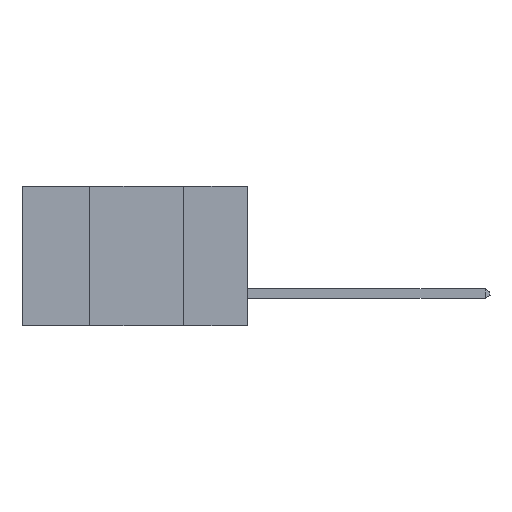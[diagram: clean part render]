
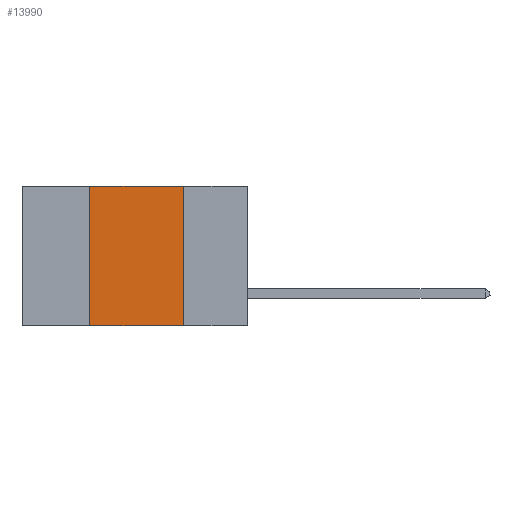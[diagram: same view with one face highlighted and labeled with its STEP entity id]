
A CAD part, left-side view. The second image highlights one B-rep face of the part: STEP entity #13990.
In plain terms, the highlighted planar face has unit normal (-1, 0, 0).
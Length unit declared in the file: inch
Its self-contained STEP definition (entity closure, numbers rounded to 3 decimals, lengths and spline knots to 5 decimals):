
#1462 = DIRECTION ( 'NONE',  ( 0., 0., -1. ) ) ;
#1663 = CARTESIAN_POINT ( 'NONE',  ( 0., 0.6, 0. ) ) ;
#2090 = DIRECTION ( 'NONE',  ( 0., -1., 0. ) ) ;
#2326 = VERTEX_POINT ( 'NONE', #18614 ) ;
#2506 = ORIENTED_EDGE ( 'NONE', *, *, #29750, .F. ) ;
#3122 = EDGE_CURVE ( 'NONE', #29241, #19191, #11850, .T. ) ;
#3670 = DIRECTION ( 'NONE',  ( 1., 0., 0. ) ) ;
#6490 = CARTESIAN_POINT ( 'NONE',  ( 0., 0.17, -0.37 ) ) ;
#7082 = LINE ( 'NONE', #9182, #16496 ) ;
#9182 = CARTESIAN_POINT ( 'NONE',  ( 0., 0.6, -0.37 ) ) ;
#10562 = CARTESIAN_POINT ( 'NONE',  ( 0., 0.6, 0. ) ) ;
#10994 = CARTESIAN_POINT ( 'NONE',  ( 0., 0.17, 0. ) ) ;
#11378 = CARTESIAN_POINT ( 'NONE',  ( 0., 0.42, -0.37 ) ) ;
#11850 = LINE ( 'NONE', #20819, #13993 ) ;
#12401 = VERTEX_POINT ( 'NONE', #6490 ) ;
#12736 = VECTOR ( 'NONE', #1462, 39.37008 ) ;
#12888 = ORIENTED_EDGE ( 'NONE', *, *, #23335, .F. ) ;
#13018 = ORIENTED_EDGE ( 'NONE', *, *, #3122, .F. ) ;
#13197 = LINE ( 'NONE', #1663, #28863 ) ;
#13990 = ADVANCED_FACE ( 'NONE', ( #22606 ), #26341, .F. ) ;
#13993 = VECTOR ( 'NONE', #25113, 39.37008 ) ;
#15661 = LINE ( 'NONE', #10994, #12736 ) ;
#16496 = VECTOR ( 'NONE', #2090, 39.37008 ) ;
#18614 = CARTESIAN_POINT ( 'NONE',  ( 0., 0.17, 0. ) ) ;
#19191 = VERTEX_POINT ( 'NONE', #22021 ) ;
#20819 = CARTESIAN_POINT ( 'NONE',  ( 0., 0.42, 0. ) ) ;
#22021 = CARTESIAN_POINT ( 'NONE',  ( 0., 0.42, 0. ) ) ;
#22606 = FACE_OUTER_BOUND ( 'NONE', #29482, .T. ) ;
#22957 = EDGE_CURVE ( 'NONE', #29241, #12401, #7082, .T. ) ;
#23335 = EDGE_CURVE ( 'NONE', #19191, #2326, #13197, .T. ) ;
#24120 = DIRECTION ( 'NONE',  ( 0., 0., -1. ) ) ;
#25113 = DIRECTION ( 'NONE',  ( 0., 0., 1. ) ) ;
#26341 = PLANE ( 'NONE',  #29440 ) ;
#26585 = ORIENTED_EDGE ( 'NONE', *, *, #22957, .T. ) ;
#28863 = VECTOR ( 'NONE', #29212, 39.37008 ) ;
#29212 = DIRECTION ( 'NONE',  ( 0., -1., 0. ) ) ;
#29241 = VERTEX_POINT ( 'NONE', #11378 ) ;
#29440 = AXIS2_PLACEMENT_3D ( 'NONE', #10562, #3670, #24120 ) ;
#29482 = EDGE_LOOP ( 'NONE', ( #2506, #12888, #13018, #26585 ) ) ;
#29750 = EDGE_CURVE ( 'NONE', #2326, #12401, #15661, .T. ) ;
